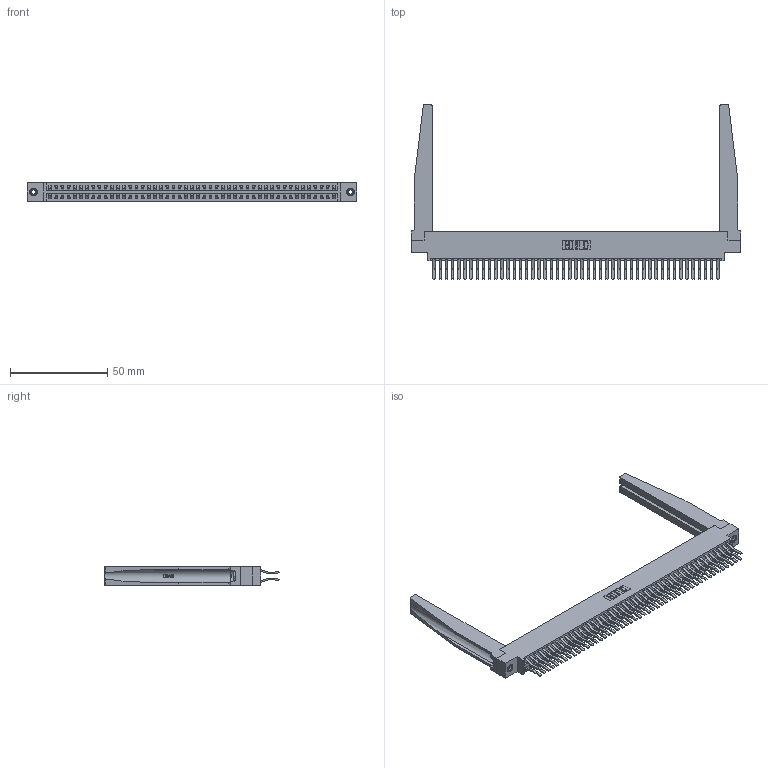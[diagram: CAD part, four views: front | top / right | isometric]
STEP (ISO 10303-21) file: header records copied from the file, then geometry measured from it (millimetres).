
FILE_DESCRIPTION (( 'STEP AP203' ), '1' );
FILE_NAME ('396-094-560-878.STEP', '2019-11-02T16:30:31', ( '' ), ( '' ), 'SwSTEP 2.0', 'SolidWorks 2016', '' );
FILE_SCHEMA (( 'CONFIG_CONTROL_DESIGN' ));
Length unit declared in the file: inch
Products named in the file (5): 345-292-001_560 Tail; 346-220-078_345-220-078; 345-250-001_345-250-001-102; 396-094-560-878; 346 Part_0.170 Offset - 0.156 Dia-TH
Assembly tree (99 placements, depth 2):
  396-094-560-878
    346 Part_0.170 Offset - 0.156 Dia-TH
    345-292-001_560 Tail  x94
    346-220-078_345-220-078  x2
    345-250-001_345-250-001-102  x2
Bounding box: 169.8 x 90.05 x 9.4 mm (x, y, z)
Volume: 23966.7 mm3; surface area: 31886.7 mm2
Topology: 99 solids, 99 shells, 5436 faces, 16083 edges, 10586 vertices
Faces by surface type: plane 3512, cylinder 1872, bspline 36, cone 12, torus 4
Entity records: 34968 total; most frequent: CARTESIAN_POINT 6695, ORIENTED_EDGE 5518, DIRECTION 4941, EDGE_CURVE 2759, VECTOR 2341, LINE 2341, VERTEX_POINT 1832, AXIS2_PLACEMENT_3D 1300
